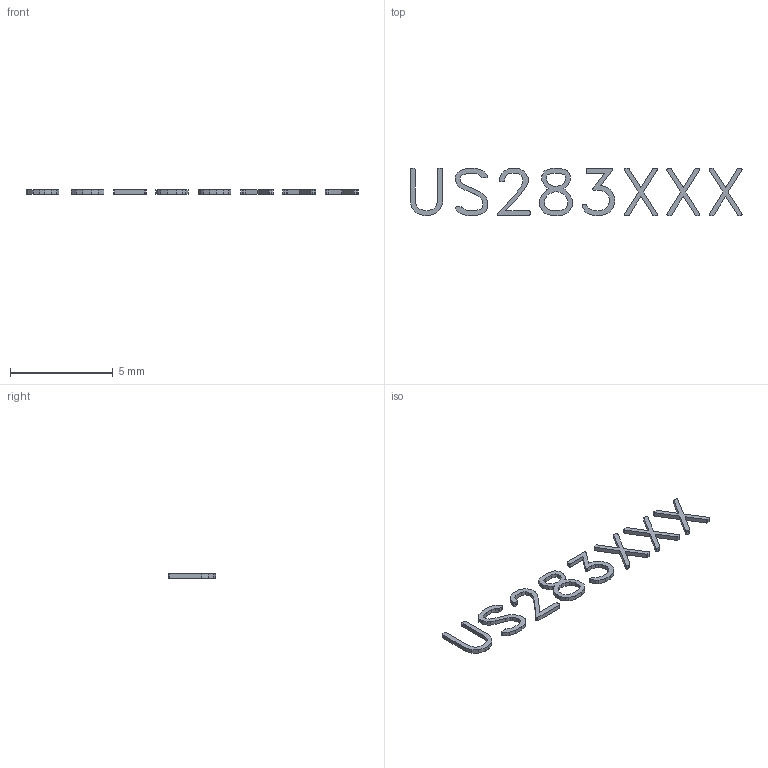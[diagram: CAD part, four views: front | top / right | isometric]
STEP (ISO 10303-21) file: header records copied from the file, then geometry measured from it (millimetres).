
FILE_DESCRIPTION (( 'STEP AP214' ), '1' );
FILE_NAME ('ENGRAVING FILL - SERIAL#.STEP', '2013-06-19T14:04:33', ( 'Asher' ), ( '' ), 'SwSTEP 2.0', 'SolidWorks 2013', '' );
FILE_SCHEMA (( 'AUTOMOTIVE_DESIGN' ));
Length unit declared in the file: millimetre
Products named in the file (1): ENGRAVING FILL - SERIAL#
Bounding box: 16.18 x 2.31 x 0.2 mm (x, y, z)
Volume: 2 mm3; surface area: 37.8 mm2
Topology: 8 solids, 8 shells, 320 faces, 912 edges, 608 vertices
Faces by surface type: plane 220, bspline 100
Entity records: 11901 total; most frequent: CARTESIAN_POINT 4141, ORIENTED_EDGE 1824, DIRECTION 1154, EDGE_CURVE 912, LINE 712, VECTOR 712, VERTEX_POINT 608, EDGE_LOOP 324
